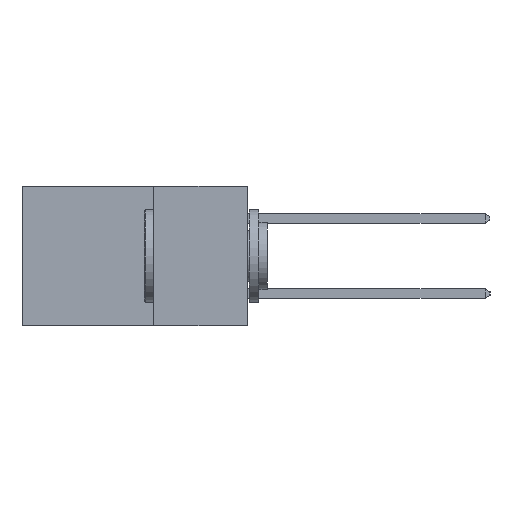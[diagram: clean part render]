
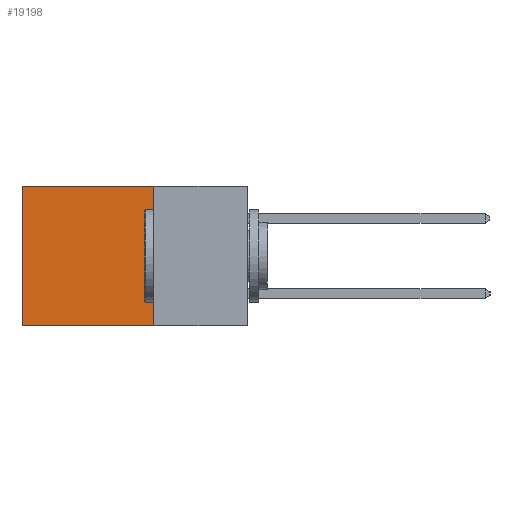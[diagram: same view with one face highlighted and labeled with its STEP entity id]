
A CAD part, left-side view. The second image highlights one B-rep face of the part: STEP entity #19198.
In plain terms, the highlighted planar face has unit normal (-1, 0, 0).
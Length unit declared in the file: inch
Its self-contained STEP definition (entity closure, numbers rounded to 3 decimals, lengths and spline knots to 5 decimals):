
#479 = LINE ( 'NONE', #8603, #17425 ) ;
#645 = DIRECTION ( 'NONE',  ( 0., 0., -1. ) ) ;
#1200 = EDGE_CURVE ( 'NONE', #4303, #17175, #18162, .T. ) ;
#2669 = DIRECTION ( 'NONE',  ( 1., 0., 0. ) ) ;
#3050 = LINE ( 'NONE', #12703, #6617 ) ;
#3295 = EDGE_CURVE ( 'NONE', #4991, #14104, #11302, .T. ) ;
#3397 = VECTOR ( 'NONE', #18253, 39.37008 ) ;
#4303 = VERTEX_POINT ( 'NONE', #4708 ) ;
#4708 = CARTESIAN_POINT ( 'NONE',  ( 0.2615, 0.25, 0. ) ) ;
#4991 = VERTEX_POINT ( 'NONE', #5623 ) ;
#5209 = ORIENTED_EDGE ( 'NONE', *, *, #1200, .T. ) ;
#5256 = ORIENTED_EDGE ( 'NONE', *, *, #9331, .F. ) ;
#5557 = EDGE_CURVE ( 'NONE', #17175, #14104, #479, .T. ) ;
#5623 = CARTESIAN_POINT ( 'NONE',  ( 0.2615, 0.25, -0.37 ) ) ;
#6617 = VECTOR ( 'NONE', #645, 39.37008 ) ;
#8089 = DIRECTION ( 'NONE',  ( 0., 0., -1. ) ) ;
#8570 = ORIENTED_EDGE ( 'NONE', *, *, #5557, .T. ) ;
#8603 = CARTESIAN_POINT ( 'NONE',  ( 0.2615, 0.6, -0.37 ) ) ;
#9331 = EDGE_CURVE ( 'NONE', #4303, #4991, #3050, .T. ) ;
#9645 = FACE_OUTER_BOUND ( 'NONE', #15865, .T. ) ;
#11302 = LINE ( 'NONE', #18237, #3397 ) ;
#12703 = CARTESIAN_POINT ( 'NONE',  ( 0.2615, 0.25, -0.37 ) ) ;
#13110 = DIRECTION ( 'NONE',  ( 0., 0., -1. ) ) ;
#13148 = AXIS2_PLACEMENT_3D ( 'NONE', #16052, #2669, #13110 ) ;
#13548 = ORIENTED_EDGE ( 'NONE', *, *, #3295, .F. ) ;
#13758 = CARTESIAN_POINT ( 'NONE',  ( 0.2615, 0.6, 0. ) ) ;
#14104 = VERTEX_POINT ( 'NONE', #17480 ) ;
#14212 = VECTOR ( 'NONE', #17426, 39.37008 ) ;
#15798 = CARTESIAN_POINT ( 'NONE',  ( 0.2615, 0.25, 0. ) ) ;
#15865 = EDGE_LOOP ( 'NONE', ( #8570, #13548, #5256, #5209 ) ) ;
#16052 = CARTESIAN_POINT ( 'NONE',  ( 0.2615, 0.25, -0.37 ) ) ;
#17175 = VERTEX_POINT ( 'NONE', #13758 ) ;
#17425 = VECTOR ( 'NONE', #8089, 39.37008 ) ;
#17426 = DIRECTION ( 'NONE',  ( 0., 1., 0. ) ) ;
#17480 = CARTESIAN_POINT ( 'NONE',  ( 0.2615, 0.6, -0.37 ) ) ;
#18162 = LINE ( 'NONE', #15798, #14212 ) ;
#18237 = CARTESIAN_POINT ( 'NONE',  ( 0.2615, 0.25, -0.37 ) ) ;
#18253 = DIRECTION ( 'NONE',  ( 0., 1., 0. ) ) ;
#19042 = PLANE ( 'NONE',  #13148 ) ;
#19198 = ADVANCED_FACE ( 'NONE', ( #9645 ), #19042, .F. ) ;
